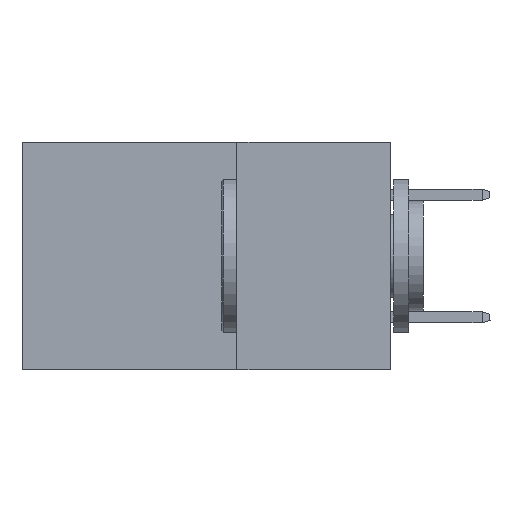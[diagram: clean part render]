
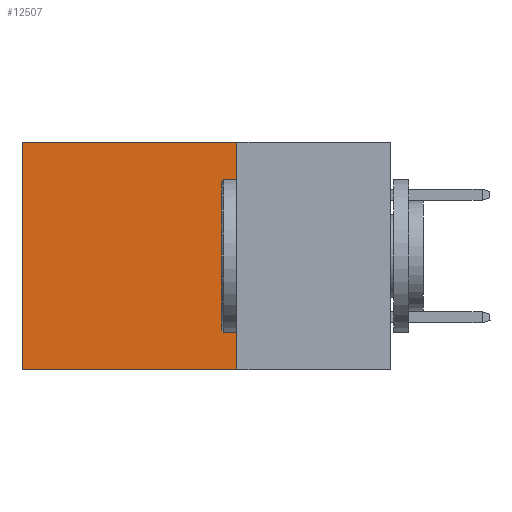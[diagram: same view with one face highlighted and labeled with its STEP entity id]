
A CAD part, left-side view. The second image highlights one B-rep face of the part: STEP entity #12507.
In plain terms, the highlighted planar face has unit normal (-1, 0, 0).
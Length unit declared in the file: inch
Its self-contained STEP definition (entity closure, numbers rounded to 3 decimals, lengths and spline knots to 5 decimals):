
#319 = EDGE_CURVE ( 'NONE', #16089, #41629, #15602, .T. ) ;
#654 = CARTESIAN_POINT ( 'NONE',  ( 0.2875, 0.25, 0. ) ) ;
#1092 = DIRECTION ( 'NONE',  ( 0., 0., -1. ) ) ;
#2099 = VERTEX_POINT ( 'NONE', #36494 ) ;
#2968 = ORIENTED_EDGE ( 'NONE', *, *, #31438, .T. ) ;
#3374 = EDGE_CURVE ( 'NONE', #9138, #2099, #34677, .T. ) ;
#3439 = ORIENTED_EDGE ( 'NONE', *, *, #3374, .F. ) ;
#4005 = DIRECTION ( 'NONE',  ( 0., 1., 0. ) ) ;
#4367 = EDGE_LOOP ( 'NONE', ( #2968, #3439, #36269, #7005 ) ) ;
#6787 = VECTOR ( 'NONE', #4005, 39.37008 ) ;
#7005 = ORIENTED_EDGE ( 'NONE', *, *, #319, .T. ) ;
#7040 = LINE ( 'NONE', #24194, #24547 ) ;
#7097 = CARTESIAN_POINT ( 'NONE',  ( 0.2875, 0.25, -0.37 ) ) ;
#9138 = VERTEX_POINT ( 'NONE', #15033 ) ;
#9530 = CARTESIAN_POINT ( 'NONE',  ( 0.2875, 0.25, 0. ) ) ;
#10396 = DIRECTION ( 'NONE',  ( 0., 0., -1. ) ) ;
#11083 = AXIS2_PLACEMENT_3D ( 'NONE', #29829, #29968, #10396 ) ;
#12507 = ADVANCED_FACE ( 'NONE', ( #27753 ), #23491, .F. ) ;
#13893 = VECTOR ( 'NONE', #14979, 39.37008 ) ;
#14385 = EDGE_CURVE ( 'NONE', #16089, #9138, #7040, .T. ) ;
#14979 = DIRECTION ( 'NONE',  ( 0., 0., -1. ) ) ;
#15033 = CARTESIAN_POINT ( 'NONE',  ( 0.2875, 0.25, -0.37 ) ) ;
#15602 = LINE ( 'NONE', #654, #6787 ) ;
#16089 = VERTEX_POINT ( 'NONE', #9530 ) ;
#17108 = DIRECTION ( 'NONE',  ( 0., 1., 0. ) ) ;
#21764 = CARTESIAN_POINT ( 'NONE',  ( 0.2875, 0.6, 0. ) ) ;
#23491 = PLANE ( 'NONE',  #11083 ) ;
#24194 = CARTESIAN_POINT ( 'NONE',  ( 0.2875, 0.25, 0. ) ) ;
#24547 = VECTOR ( 'NONE', #1092, 39.37008 ) ;
#26157 = VECTOR ( 'NONE', #17108, 39.37008 ) ;
#27753 = FACE_OUTER_BOUND ( 'NONE', #4367, .T. ) ;
#29829 = CARTESIAN_POINT ( 'NONE',  ( 0.2875, 0.25, 0. ) ) ;
#29968 = DIRECTION ( 'NONE',  ( 1., 0., 0. ) ) ;
#30208 = LINE ( 'NONE', #34421, #13893 ) ;
#31438 = EDGE_CURVE ( 'NONE', #41629, #2099, #30208, .T. ) ;
#34421 = CARTESIAN_POINT ( 'NONE',  ( 0.2875, 0.6, 0. ) ) ;
#34677 = LINE ( 'NONE', #7097, #26157 ) ;
#36269 = ORIENTED_EDGE ( 'NONE', *, *, #14385, .F. ) ;
#36494 = CARTESIAN_POINT ( 'NONE',  ( 0.2875, 0.6, -0.37 ) ) ;
#41629 = VERTEX_POINT ( 'NONE', #21764 ) ;
